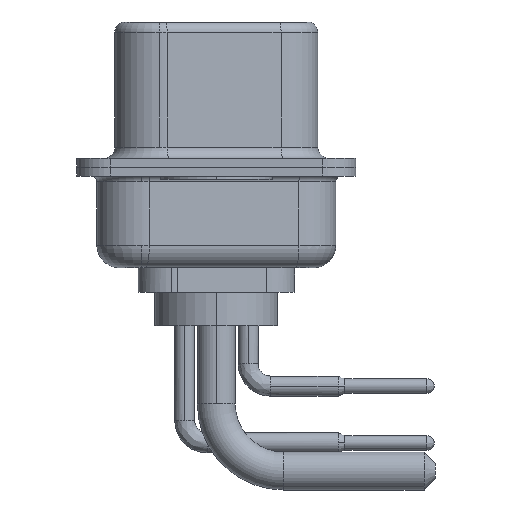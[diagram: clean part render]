
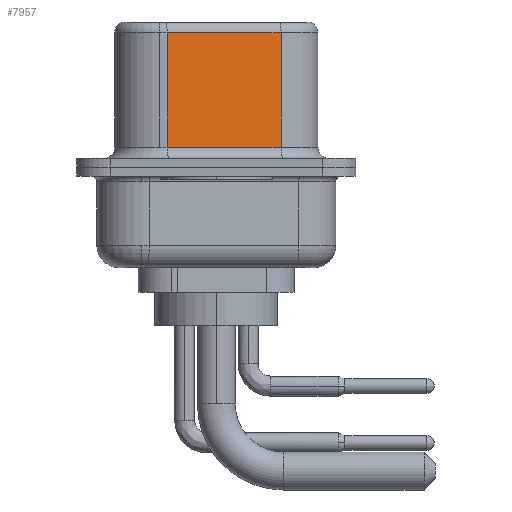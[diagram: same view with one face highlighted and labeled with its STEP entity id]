
A CAD part, left-side view. The second image highlights one B-rep face of the part: STEP entity #7957.
In plain terms, the highlighted planar face has unit normal (-0.985, -0.174, 0).
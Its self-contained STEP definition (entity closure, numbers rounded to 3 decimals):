
#49 = EDGE_CURVE ( 'NONE', #15496, #12685, #4037, .T. ) ;
#321 = EDGE_CURVE ( 'NONE', #14521, #14060, #3437, .T. ) ;
#658 = VECTOR ( 'NONE', #744, 1000. ) ;
#744 = DIRECTION ( 'NONE',  ( 0.174, -0.985, 0. ) ) ;
#1888 = DIRECTION ( 'NONE',  ( 0., 0., -1. ) ) ;
#3056 = EDGE_CURVE ( 'NONE', #12685, #14060, #14021, .T. ) ;
#3437 = LINE ( 'NONE', #18068, #5205 ) ;
#3490 = CARTESIAN_POINT ( 'NONE',  ( 3.655, 2.203, 6.02 ) ) ;
#3848 = DIRECTION ( 'NONE',  ( 0., 0., -1. ) ) ;
#4037 = LINE ( 'NONE', #8586, #18737 ) ;
#4172 = CARTESIAN_POINT ( 'NONE',  ( 4.555, -2.897, 0.9 ) ) ;
#5205 = VECTOR ( 'NONE', #1888, 1000. ) ;
#5419 = FACE_OUTER_BOUND ( 'NONE', #15981, .T. ) ;
#6174 = CARTESIAN_POINT ( 'NONE',  ( 4.555, -2.897, 6.02 ) ) ;
#6858 = EDGE_CURVE ( 'NONE', #14521, #15496, #12109, .T. ) ;
#7957 = ADVANCED_FACE ( 'NONE', ( #5419 ), #10262, .F. ) ;
#8586 = CARTESIAN_POINT ( 'NONE',  ( 3.655, 2.203, 6.52 ) ) ;
#9104 = ORIENTED_EDGE ( 'NONE', *, *, #6858, .T. ) ;
#9818 = VECTOR ( 'NONE', #10565, 1000. ) ;
#10060 = DIRECTION ( 'NONE',  ( 0.985, 0.174, 0. ) ) ;
#10262 = PLANE ( 'NONE',  #14204 ) ;
#10565 = DIRECTION ( 'NONE',  ( -0.174, 0.985, 0. ) ) ;
#10620 = CARTESIAN_POINT ( 'NONE',  ( 4.555, -2.897, 6.02 ) ) ;
#12109 = LINE ( 'NONE', #6174, #9818 ) ;
#12355 = CARTESIAN_POINT ( 'NONE',  ( 4.555, -2.897, 0.9 ) ) ;
#12685 = VERTEX_POINT ( 'NONE', #14244 ) ;
#12726 = ORIENTED_EDGE ( 'NONE', *, *, #321, .F. ) ;
#14021 = LINE ( 'NONE', #12355, #658 ) ;
#14060 = VERTEX_POINT ( 'NONE', #4172 ) ;
#14204 = AXIS2_PLACEMENT_3D ( 'NONE', #14720, #10060, #17254 ) ;
#14244 = CARTESIAN_POINT ( 'NONE',  ( 3.655, 2.203, 0.9 ) ) ;
#14521 = VERTEX_POINT ( 'NONE', #10620 ) ;
#14720 = CARTESIAN_POINT ( 'NONE',  ( 4.555, -2.897, 6.52 ) ) ;
#15496 = VERTEX_POINT ( 'NONE', #3490 ) ;
#15633 = ORIENTED_EDGE ( 'NONE', *, *, #49, .T. ) ;
#15981 = EDGE_LOOP ( 'NONE', ( #12726, #9104, #15633, #16255 ) ) ;
#16255 = ORIENTED_EDGE ( 'NONE', *, *, #3056, .T. ) ;
#17254 = DIRECTION ( 'NONE',  ( -0.174, 0.985, 0. ) ) ;
#18068 = CARTESIAN_POINT ( 'NONE',  ( 4.555, -2.897, 6.52 ) ) ;
#18737 = VECTOR ( 'NONE', #3848, 1000. ) ;
